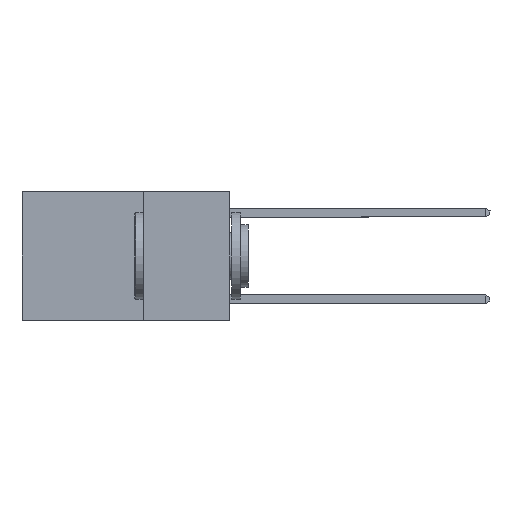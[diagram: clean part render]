
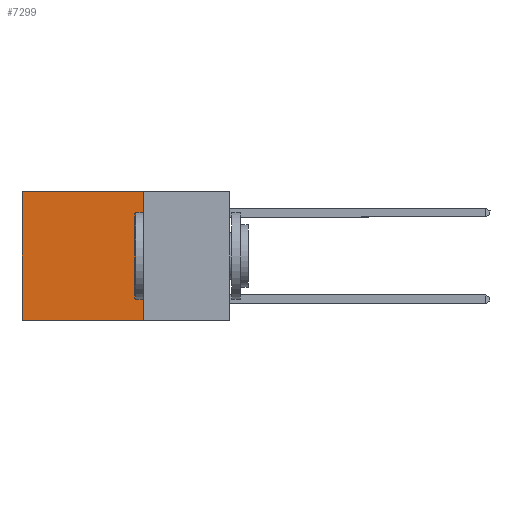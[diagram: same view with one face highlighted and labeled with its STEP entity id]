
A CAD part, left-side view. The second image highlights one B-rep face of the part: STEP entity #7299.
In plain terms, the highlighted planar face has unit normal (-1, 0, 0).
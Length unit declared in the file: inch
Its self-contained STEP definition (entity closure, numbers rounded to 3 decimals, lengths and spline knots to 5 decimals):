
#259 = DIRECTION ( 'NONE',  ( 0., 0., -1. ) ) ;
#265 = ORIENTED_EDGE ( 'NONE', *, *, #11196, .T. ) ;
#619 = PLANE ( 'NONE',  #12858 ) ;
#1429 = VECTOR ( 'NONE', #10776, 39.37008 ) ;
#1637 = ORIENTED_EDGE ( 'NONE', *, *, #11722, .T. ) ;
#2023 = CARTESIAN_POINT ( 'NONE',  ( 0.2625, 0.6, 0. ) ) ;
#2072 = LINE ( 'NONE', #12693, #1429 ) ;
#2226 = VECTOR ( 'NONE', #12517, 39.37008 ) ;
#2700 = DIRECTION ( 'NONE',  ( 0., 0., -1. ) ) ;
#3408 = VERTEX_POINT ( 'NONE', #8216 ) ;
#3782 = ORIENTED_EDGE ( 'NONE', *, *, #10157, .F. ) ;
#4366 = LINE ( 'NONE', #8840, #9458 ) ;
#4449 = VERTEX_POINT ( 'NONE', #2023 ) ;
#4760 = CARTESIAN_POINT ( 'NONE',  ( 0.2625, 0.25, 0. ) ) ;
#4809 = DIRECTION ( 'NONE',  ( 0., 0., -1. ) ) ;
#5522 = CARTESIAN_POINT ( 'NONE',  ( 0.2625, 0.25, 0. ) ) ;
#6350 = CARTESIAN_POINT ( 'NONE',  ( 0.2625, 0.6, -0.37 ) ) ;
#7004 = FACE_OUTER_BOUND ( 'NONE', #12242, .T. ) ;
#7120 = LINE ( 'NONE', #7414, #9510 ) ;
#7299 = ADVANCED_FACE ( 'NONE', ( #7004 ), #619, .F. ) ;
#7414 = CARTESIAN_POINT ( 'NONE',  ( 0.2625, 0.25, 0. ) ) ;
#7715 = CARTESIAN_POINT ( 'NONE',  ( 0.2625, 0.25, 0. ) ) ;
#8216 = CARTESIAN_POINT ( 'NONE',  ( 0.2625, 0.25, -0.37 ) ) ;
#8225 = ORIENTED_EDGE ( 'NONE', *, *, #9171, .F. ) ;
#8737 = DIRECTION ( 'NONE',  ( 1., 0., 0. ) ) ;
#8840 = CARTESIAN_POINT ( 'NONE',  ( 0.2625, 0.6, 0. ) ) ;
#9109 = VERTEX_POINT ( 'NONE', #6350 ) ;
#9171 = EDGE_CURVE ( 'NONE', #11158, #3408, #7120, .T. ) ;
#9458 = VECTOR ( 'NONE', #4809, 39.37008 ) ;
#9510 = VECTOR ( 'NONE', #259, 39.37008 ) ;
#9932 = LINE ( 'NONE', #5522, #2226 ) ;
#10157 = EDGE_CURVE ( 'NONE', #3408, #9109, #2072, .T. ) ;
#10776 = DIRECTION ( 'NONE',  ( 0., 1., 0. ) ) ;
#11158 = VERTEX_POINT ( 'NONE', #4760 ) ;
#11196 = EDGE_CURVE ( 'NONE', #4449, #9109, #4366, .T. ) ;
#11722 = EDGE_CURVE ( 'NONE', #11158, #4449, #9932, .T. ) ;
#12242 = EDGE_LOOP ( 'NONE', ( #265, #3782, #8225, #1637 ) ) ;
#12517 = DIRECTION ( 'NONE',  ( 0., 1., 0. ) ) ;
#12693 = CARTESIAN_POINT ( 'NONE',  ( 0.2625, 0.25, -0.37 ) ) ;
#12858 = AXIS2_PLACEMENT_3D ( 'NONE', #7715, #8737, #2700 ) ;
